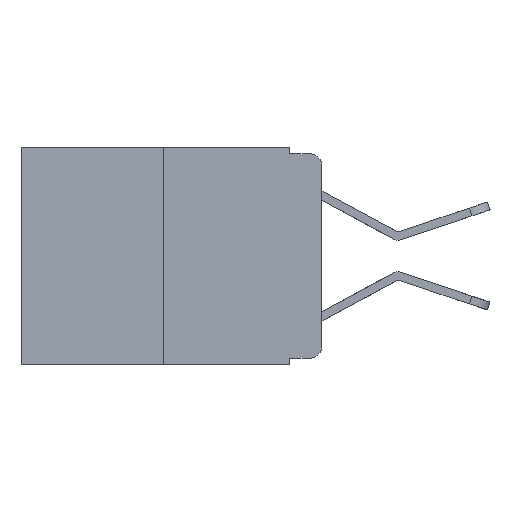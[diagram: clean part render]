
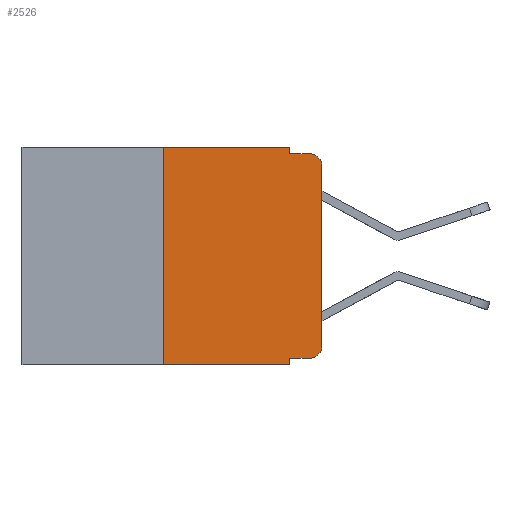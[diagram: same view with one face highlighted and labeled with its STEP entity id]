
A CAD part, left-side view. The second image highlights one B-rep face of the part: STEP entity #2526.
In plain terms, the highlighted planar face has unit normal (-1, 0, 0).
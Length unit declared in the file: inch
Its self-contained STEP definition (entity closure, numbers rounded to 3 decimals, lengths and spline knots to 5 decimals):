
#411 = EDGE_CURVE ( 'NONE', #7579, #6373, #16813, .T. ) ;
#550 = EDGE_CURVE ( 'NONE', #11915, #6266, #4944, .T. ) ;
#815 = LINE ( 'NONE', #8060, #5026 ) ;
#1068 = CARTESIAN_POINT ( 'NONE',  ( 0., 0.051, 0. ) ) ;
#1218 = CIRCLE ( 'NONE', #13191, 0.02 ) ;
#1918 = LINE ( 'NONE', #11804, #15425 ) ;
#1949 = DIRECTION ( 'NONE',  ( 0., -1., 0. ) ) ;
#1985 = DIRECTION ( 'NONE',  ( -1., 0., 0. ) ) ;
#2526 = ADVANCED_FACE ( 'NONE', ( #7634 ), #10282, .F. ) ;
#2579 = ORIENTED_EDGE ( 'NONE', *, *, #9817, .F. ) ;
#2732 = DIRECTION ( 'NONE',  ( 0., 0., 1. ) ) ;
#2823 = EDGE_CURVE ( 'NONE', #3743, #12259, #12817, .T. ) ;
#3183 = CARTESIAN_POINT ( 'NONE',  ( 0., 0.473, 0. ) ) ;
#3281 = VECTOR ( 'NONE', #2732, 39.37008 ) ;
#3396 = DIRECTION ( 'NONE',  ( 0., 0., -1. ) ) ;
#3654 = EDGE_CURVE ( 'NONE', #12259, #15413, #10527, .T. ) ;
#3679 = LINE ( 'NONE', #15591, #14015 ) ;
#3700 = VERTEX_POINT ( 'NONE', #13474 ) ;
#3743 = VERTEX_POINT ( 'NONE', #13109 ) ;
#4403 = CARTESIAN_POINT ( 'NONE',  ( 0., 0., -0.03 ) ) ;
#4777 = CARTESIAN_POINT ( 'NONE',  ( 0., 0.473, -0.343 ) ) ;
#4818 = CARTESIAN_POINT ( 'NONE',  ( 0., 0., -0.313 ) ) ;
#4944 = LINE ( 'NONE', #11603, #10852 ) ;
#5026 = VECTOR ( 'NONE', #9434, 39.37008 ) ;
#5084 = AXIS2_PLACEMENT_3D ( 'NONE', #10531, #1985, #3396 ) ;
#5525 = EDGE_CURVE ( 'NONE', #15413, #6266, #1218, .T. ) ;
#5592 = VERTEX_POINT ( 'NONE', #12849 ) ;
#6020 = ORIENTED_EDGE ( 'NONE', *, *, #10897, .F. ) ;
#6204 = VECTOR ( 'NONE', #16548, 39.37008 ) ;
#6266 = VERTEX_POINT ( 'NONE', #11590 ) ;
#6314 = AXIS2_PLACEMENT_3D ( 'NONE', #14032, #15957, #16793 ) ;
#6373 = VERTEX_POINT ( 'NONE', #9222 ) ;
#6786 = ORIENTED_EDGE ( 'NONE', *, *, #550, .F. ) ;
#7002 = ORIENTED_EDGE ( 'NONE', *, *, #5525, .T. ) ;
#7323 = ORIENTED_EDGE ( 'NONE', *, *, #3654, .T. ) ;
#7386 = ORIENTED_EDGE ( 'NONE', *, *, #411, .F. ) ;
#7579 = VERTEX_POINT ( 'NONE', #10638 ) ;
#7634 = FACE_OUTER_BOUND ( 'NONE', #12319, .T. ) ;
#7650 = ORIENTED_EDGE ( 'NONE', *, *, #11001, .T. ) ;
#7837 = ORIENTED_EDGE ( 'NONE', *, *, #11881, .F. ) ;
#8060 = CARTESIAN_POINT ( 'NONE',  ( 0., 0.051, 0. ) ) ;
#8117 = CARTESIAN_POINT ( 'NONE',  ( 0., 0.051, -0.01 ) ) ;
#8198 = CARTESIAN_POINT ( 'NONE',  ( 0., 0.051, -0.333 ) ) ;
#8497 = ORIENTED_EDGE ( 'NONE', *, *, #2823, .T. ) ;
#9003 = VECTOR ( 'NONE', #1949, 39.37008 ) ;
#9209 = DIRECTION ( 'NONE',  ( 0., -1., 0. ) ) ;
#9222 = CARTESIAN_POINT ( 'NONE',  ( 0., 0.051, 0. ) ) ;
#9434 = DIRECTION ( 'NONE',  ( 0., 0., -1. ) ) ;
#9443 = LINE ( 'NONE', #4777, #9003 ) ;
#9817 = EDGE_CURVE ( 'NONE', #6373, #11915, #10738, .T. ) ;
#9928 = DIRECTION ( 'NONE',  ( 0., 0., -1. ) ) ;
#10282 = PLANE ( 'NONE',  #6314 ) ;
#10527 = LINE ( 'NONE', #12915, #3281 ) ;
#10531 = CARTESIAN_POINT ( 'NONE',  ( 0., 0.02, -0.313 ) ) ;
#10638 = CARTESIAN_POINT ( 'NONE',  ( 0., 0.25, 0. ) ) ;
#10696 = DIRECTION ( 'NONE',  ( 0., 0., -1. ) ) ;
#10738 = LINE ( 'NONE', #1068, #14252 ) ;
#10852 = VECTOR ( 'NONE', #16827, 39.37008 ) ;
#10897 = EDGE_CURVE ( 'NONE', #5592, #7579, #3679, .T. ) ;
#11001 = EDGE_CURVE ( 'NONE', #16909, #3743, #1918, .T. ) ;
#11177 = DIRECTION ( 'NONE',  ( -1., 0., 0. ) ) ;
#11590 = CARTESIAN_POINT ( 'NONE',  ( 0., 0.02, -0.01 ) ) ;
#11603 = CARTESIAN_POINT ( 'NONE',  ( 0., 0.051, -0.01 ) ) ;
#11804 = CARTESIAN_POINT ( 'NONE',  ( 0., 0.051, -0.333 ) ) ;
#11881 = EDGE_CURVE ( 'NONE', #16909, #3700, #815, .T. ) ;
#11915 = VERTEX_POINT ( 'NONE', #8117 ) ;
#12259 = VERTEX_POINT ( 'NONE', #4818 ) ;
#12319 = EDGE_LOOP ( 'NONE', ( #7323, #7002, #6786, #2579, #7386, #6020, #14277, #7837, #7650, #8497 ) ) ;
#12817 = CIRCLE ( 'NONE', #5084, 0.02 ) ;
#12849 = CARTESIAN_POINT ( 'NONE',  ( 0., 0.25, -0.343 ) ) ;
#12915 = CARTESIAN_POINT ( 'NONE',  ( 0., 0., 0. ) ) ;
#12997 = CARTESIAN_POINT ( 'NONE',  ( 0., 0.02, -0.03 ) ) ;
#13109 = CARTESIAN_POINT ( 'NONE',  ( 0., 0.02, -0.333 ) ) ;
#13191 = AXIS2_PLACEMENT_3D ( 'NONE', #12997, #11177, #9928 ) ;
#13474 = CARTESIAN_POINT ( 'NONE',  ( 0., 0.051, -0.343 ) ) ;
#13517 = EDGE_CURVE ( 'NONE', #5592, #3700, #9443, .T. ) ;
#14015 = VECTOR ( 'NONE', #16855, 39.37008 ) ;
#14032 = CARTESIAN_POINT ( 'NONE',  ( 0., 0.473, 0. ) ) ;
#14252 = VECTOR ( 'NONE', #10696, 39.37008 ) ;
#14277 = ORIENTED_EDGE ( 'NONE', *, *, #13517, .T. ) ;
#15413 = VERTEX_POINT ( 'NONE', #4403 ) ;
#15425 = VECTOR ( 'NONE', #9209, 39.37008 ) ;
#15591 = CARTESIAN_POINT ( 'NONE',  ( 0., 0.25, 0. ) ) ;
#15957 = DIRECTION ( 'NONE',  ( 1., 0., 0. ) ) ;
#16548 = DIRECTION ( 'NONE',  ( 0., -1., 0. ) ) ;
#16793 = DIRECTION ( 'NONE',  ( 0., 0., -1. ) ) ;
#16813 = LINE ( 'NONE', #3183, #6204 ) ;
#16827 = DIRECTION ( 'NONE',  ( 0., -1., 0. ) ) ;
#16855 = DIRECTION ( 'NONE',  ( 0., 0., 1. ) ) ;
#16909 = VERTEX_POINT ( 'NONE', #8198 ) ;
